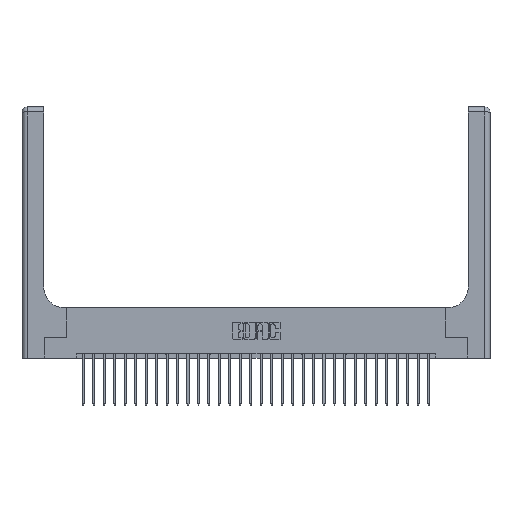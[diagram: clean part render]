
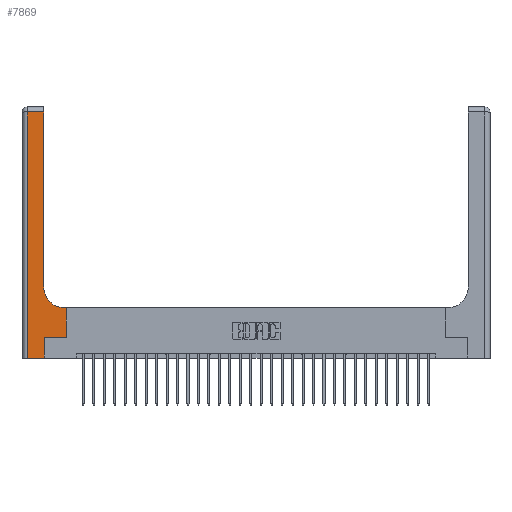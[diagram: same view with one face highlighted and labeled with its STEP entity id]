
A CAD part, top view. The second image highlights one B-rep face of the part: STEP entity #7869.
In plain terms, the highlighted planar face has unit normal (0, 0, 1).
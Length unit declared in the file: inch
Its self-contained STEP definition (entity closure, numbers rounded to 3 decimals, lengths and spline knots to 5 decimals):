
#791 = CARTESIAN_POINT ( 'NONE',  ( 0., 0., 0.37 ) ) ;
#847 = EDGE_CURVE ( 'NONE', #15756, #1079, #7424, .T. ) ;
#1079 = VERTEX_POINT ( 'NONE', #8716 ) ;
#1469 = DIRECTION ( 'NONE',  ( 0., -1., 0. ) ) ;
#1765 = CARTESIAN_POINT ( 'NONE',  ( 0.265, 0., 0.37 ) ) ;
#2345 = DIRECTION ( 'NONE',  ( 1., 0., 0. ) ) ;
#2446 = CARTESIAN_POINT ( 'NONE',  ( 0.51, 0.85, 0.37 ) ) ;
#3058 = CARTESIAN_POINT ( 'NONE',  ( 0.26, 0.85, 0.37 ) ) ;
#3452 = DIRECTION ( 'NONE',  ( 0., 1., 0. ) ) ;
#3566 = CARTESIAN_POINT ( 'NONE',  ( 0., 2.94, 0.37 ) ) ;
#4501 = CARTESIAN_POINT ( 'NONE',  ( 0.265, 0.25, 0.37 ) ) ;
#4637 = VERTEX_POINT ( 'NONE', #16155 ) ;
#4862 = DIRECTION ( 'NONE',  ( 1., 0., 0. ) ) ;
#5683 = DIRECTION ( 'NONE',  ( 0., 1., 0. ) ) ;
#5776 = DIRECTION ( 'NONE',  ( -1., 0., 0. ) ) ;
#5807 = VECTOR ( 'NONE', #3452, 39.37008 ) ;
#6505 = VERTEX_POINT ( 'NONE', #26414 ) ;
#6693 = VECTOR ( 'NONE', #7752, 39.37008 ) ;
#7314 = ORIENTED_EDGE ( 'NONE', *, *, #9120, .T. ) ;
#7424 = LINE ( 'NONE', #4501, #20488 ) ;
#7431 = EDGE_LOOP ( 'NONE', ( #14379, #27479, #27697, #27155, #7314, #9055, #26505, #9402, #28460 ) ) ;
#7752 = DIRECTION ( 'NONE',  ( 0., 1., 0. ) ) ;
#7869 = ADVANCED_FACE ( 'NONE', ( #9575 ), #25512, .F. ) ;
#8166 = CARTESIAN_POINT ( 'NONE',  ( 0.26, 2.94, 0.37 ) ) ;
#8508 = VERTEX_POINT ( 'NONE', #20395 ) ;
#8716 = CARTESIAN_POINT ( 'NONE',  ( 0.528, 0.25, 0.37 ) ) ;
#9055 = ORIENTED_EDGE ( 'NONE', *, *, #847, .T. ) ;
#9120 = EDGE_CURVE ( 'NONE', #27751, #15756, #11454, .T. ) ;
#9402 = ORIENTED_EDGE ( 'NONE', *, *, #11712, .T. ) ;
#9575 = FACE_OUTER_BOUND ( 'NONE', #7431, .T. ) ;
#9750 = EDGE_CURVE ( 'NONE', #15225, #11287, #11433, .T. ) ;
#10110 = CARTESIAN_POINT ( 'NONE',  ( 0.26, 0.6, 0.37 ) ) ;
#10415 = DIRECTION ( 'NONE',  ( -1., 0., 0. ) ) ;
#11023 = AXIS2_PLACEMENT_3D ( 'NONE', #21192, #12512, #10415 ) ;
#11155 = LINE ( 'NONE', #25972, #18064 ) ;
#11287 = VERTEX_POINT ( 'NONE', #8166 ) ;
#11325 = LINE ( 'NONE', #791, #20304 ) ;
#11433 = LINE ( 'NONE', #12377, #12117 ) ;
#11454 = LINE ( 'NONE', #16094, #6693 ) ;
#11571 = EDGE_CURVE ( 'NONE', #8508, #27751, #11325, .T. ) ;
#11712 = EDGE_CURVE ( 'NONE', #4637, #20982, #26513, .T. ) ;
#12117 = VECTOR ( 'NONE', #5683, 39.37008 ) ;
#12377 = CARTESIAN_POINT ( 'NONE',  ( 0.26, 3., 0.37 ) ) ;
#12512 = DIRECTION ( 'NONE',  ( 0., 0., -1. ) ) ;
#13794 = AXIS2_PLACEMENT_3D ( 'NONE', #2446, #15502, #2345 ) ;
#14194 = EDGE_CURVE ( 'NONE', #11287, #6505, #20859, .T. ) ;
#14379 = ORIENTED_EDGE ( 'NONE', *, *, #9750, .T. ) ;
#14521 = DIRECTION ( 'NONE',  ( -1., 0., 0. ) ) ;
#15098 = VECTOR ( 'NONE', #14521, 39.37008 ) ;
#15225 = VERTEX_POINT ( 'NONE', #3058 ) ;
#15502 = DIRECTION ( 'NONE',  ( 0., 0., -1. ) ) ;
#15756 = VERTEX_POINT ( 'NONE', #17259 ) ;
#16022 = CARTESIAN_POINT ( 'NONE',  ( 0.51, 0.6, 0.37 ) ) ;
#16094 = CARTESIAN_POINT ( 'NONE',  ( 0.265, 0., 0.37 ) ) ;
#16155 = CARTESIAN_POINT ( 'NONE',  ( 0.528, 0.6, 0.37 ) ) ;
#17125 = EDGE_CURVE ( 'NONE', #6505, #8508, #11155, .T. ) ;
#17259 = CARTESIAN_POINT ( 'NONE',  ( 0.265, 0.25, 0.37 ) ) ;
#18064 = VECTOR ( 'NONE', #1469, 39.37008 ) ;
#18210 = LINE ( 'NONE', #22864, #5807 ) ;
#19897 = DIRECTION ( 'NONE',  ( 1., 0., 0. ) ) ;
#20282 = CIRCLE ( 'NONE', #13794, 0.25 ) ;
#20304 = VECTOR ( 'NONE', #4862, 39.37008 ) ;
#20395 = CARTESIAN_POINT ( 'NONE',  ( 0.06, 0., 0.37 ) ) ;
#20488 = VECTOR ( 'NONE', #19897, 39.37008 ) ;
#20859 = LINE ( 'NONE', #3566, #24604 ) ;
#20982 = VERTEX_POINT ( 'NONE', #16022 ) ;
#21192 = CARTESIAN_POINT ( 'NONE',  ( 0., 3., 0.37 ) ) ;
#21498 = EDGE_CURVE ( 'NONE', #1079, #4637, #18210, .T. ) ;
#22864 = CARTESIAN_POINT ( 'NONE',  ( 0.528, 0.25, 0.37 ) ) ;
#24604 = VECTOR ( 'NONE', #5776, 39.37008 ) ;
#25512 = PLANE ( 'NONE',  #11023 ) ;
#25972 = CARTESIAN_POINT ( 'NONE',  ( 0.06, 3., 0.37 ) ) ;
#26414 = CARTESIAN_POINT ( 'NONE',  ( 0.06, 2.94, 0.37 ) ) ;
#26505 = ORIENTED_EDGE ( 'NONE', *, *, #21498, .T. ) ;
#26513 = LINE ( 'NONE', #10110, #15098 ) ;
#27155 = ORIENTED_EDGE ( 'NONE', *, *, #11571, .T. ) ;
#27479 = ORIENTED_EDGE ( 'NONE', *, *, #14194, .T. ) ;
#27697 = ORIENTED_EDGE ( 'NONE', *, *, #17125, .T. ) ;
#27751 = VERTEX_POINT ( 'NONE', #1765 ) ;
#27947 = EDGE_CURVE ( 'NONE', #20982, #15225, #20282, .T. ) ;
#28460 = ORIENTED_EDGE ( 'NONE', *, *, #27947, .T. ) ;
